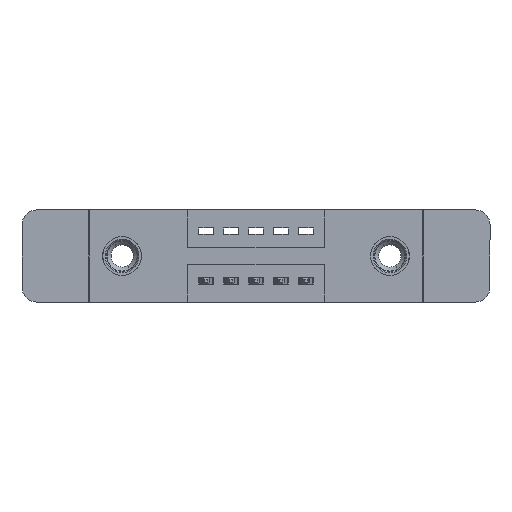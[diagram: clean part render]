
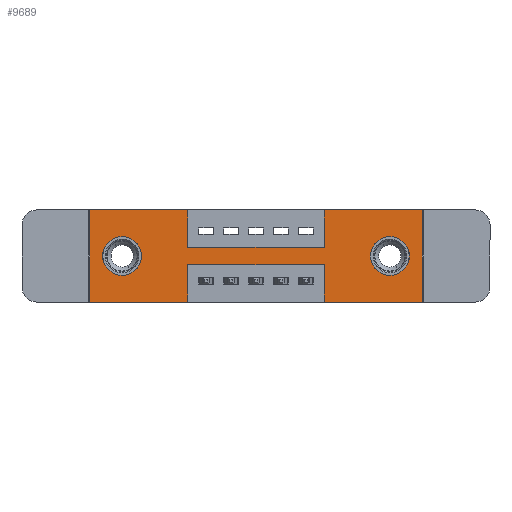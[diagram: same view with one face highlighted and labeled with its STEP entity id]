
A CAD part, front view. The second image highlights one B-rep face of the part: STEP entity #9689.
In plain terms, the highlighted planar face has unit normal (0, -1, 0).
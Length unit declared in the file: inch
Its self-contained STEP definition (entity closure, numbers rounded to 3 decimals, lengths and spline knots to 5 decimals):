
#65 = ORIENTED_EDGE ( 'NONE', *, *, #8855, .F. ) ;
#238 = CARTESIAN_POINT ( 'NONE',  ( 0.3925, 0., -0.15 ) ) ;
#316 = EDGE_CURVE ( 'NONE', #12437, #9325, #3677, .T. ) ;
#398 = CARTESIAN_POINT ( 'NONE',  ( 0.13, 0., -0.107 ) ) ;
#513 = ORIENTED_EDGE ( 'NONE', *, *, #13121, .F. ) ;
#515 = DIRECTION ( 'NONE',  ( 0., -1., 0. ) ) ;
#548 = AXIS2_PLACEMENT_3D ( 'NONE', #12380, #5952, #3836 ) ;
#571 = DIRECTION ( 'NONE',  ( 0., 0., -1. ) ) ;
#589 = CARTESIAN_POINT ( 'NONE',  ( 0., 0., -0.37 ) ) ;
#710 = VERTEX_POINT ( 'NONE', #9934 ) ;
#1002 = FACE_BOUND ( 'NONE', #13647, .T. ) ;
#1072 = VECTOR ( 'NONE', #3995, 39.37008 ) ;
#1135 = EDGE_CURVE ( 'NONE', #1375, #8630, #1816, .T. ) ;
#1375 = VERTEX_POINT ( 'NONE', #13892 ) ;
#1467 = CARTESIAN_POINT ( 'NONE',  ( 0., 0., 0. ) ) ;
#1702 = VERTEX_POINT ( 'NONE', #7145 ) ;
#1800 = CARTESIAN_POINT ( 'NONE',  ( 0., 0., -0.37 ) ) ;
#1816 = LINE ( 'NONE', #9152, #13083 ) ;
#1893 = CIRCLE ( 'NONE', #8534, 0.078 ) ;
#1899 = ORIENTED_EDGE ( 'NONE', *, *, #11169, .F. ) ;
#1965 = CARTESIAN_POINT ( 'NONE',  ( 0., 0., 0. ) ) ;
#1981 = CARTESIAN_POINT ( 'NONE',  ( 0.3925, 0., -0.37 ) ) ;
#2000 = CARTESIAN_POINT ( 'NONE',  ( 0.3925, 0., 0. ) ) ;
#2028 = ORIENTED_EDGE ( 'NONE', *, *, #316, .T. ) ;
#2043 = ORIENTED_EDGE ( 'NONE', *, *, #1135, .F. ) ;
#2092 = DIRECTION ( 'NONE',  ( 0., 0., -1. ) ) ;
#2189 = VERTEX_POINT ( 'NONE', #7234 ) ;
#2314 = CARTESIAN_POINT ( 'NONE',  ( 0., 0., 0. ) ) ;
#2426 = VECTOR ( 'NONE', #8026, 39.37008 ) ;
#2436 = EDGE_CURVE ( 'NONE', #1702, #11896, #8684, .T. ) ;
#2542 = EDGE_CURVE ( 'NONE', #710, #1375, #6013, .T. ) ;
#2558 = CIRCLE ( 'NONE', #548, 0.078 ) ;
#2663 = PLANE ( 'NONE',  #7568 ) ;
#2978 = VERTEX_POINT ( 'NONE', #398 ) ;
#3062 = ORIENTED_EDGE ( 'NONE', *, *, #13079, .F. ) ;
#3138 = DIRECTION ( 'NONE',  ( 0., 0., -1. ) ) ;
#3182 = VERTEX_POINT ( 'NONE', #5188 ) ;
#3246 = VECTOR ( 'NONE', #9193, 39.37008 ) ;
#3677 = CIRCLE ( 'NONE', #13862, 0.078 ) ;
#3764 = CARTESIAN_POINT ( 'NONE',  ( 0., 0., -0.37 ) ) ;
#3794 = CARTESIAN_POINT ( 'NONE',  ( 0.9425, 0., 0. ) ) ;
#3815 = CARTESIAN_POINT ( 'NONE',  ( 1.205, 0., -0.185 ) ) ;
#3836 = DIRECTION ( 'NONE',  ( 0., 0., 1. ) ) ;
#3938 = CIRCLE ( 'NONE', #5187, 0.078 ) ;
#3967 = CARTESIAN_POINT ( 'NONE',  ( 0.3925, 0., -0.22 ) ) ;
#3990 = LINE ( 'NONE', #2314, #9192 ) ;
#3995 = DIRECTION ( 'NONE',  ( -1., 0., 0. ) ) ;
#3996 = VERTEX_POINT ( 'NONE', #12141 ) ;
#4077 = EDGE_CURVE ( 'NONE', #13248, #2978, #2558, .T. ) ;
#4109 = VECTOR ( 'NONE', #4788, 39.37008 ) ;
#4272 = EDGE_CURVE ( 'NONE', #2978, #13248, #1893, .T. ) ;
#4352 = EDGE_CURVE ( 'NONE', #9325, #12437, #3938, .T. ) ;
#4690 = VECTOR ( 'NONE', #12716, 39.37008 ) ;
#4745 = CARTESIAN_POINT ( 'NONE',  ( 0.13, 0., -0.185 ) ) ;
#4788 = DIRECTION ( 'NONE',  ( 0., 0., 1. ) ) ;
#4891 = DIRECTION ( 'NONE',  ( 0., 1., 0. ) ) ;
#4926 = CARTESIAN_POINT ( 'NONE',  ( 1.205, 0., -0.185 ) ) ;
#4978 = VECTOR ( 'NONE', #9907, 39.37008 ) ;
#5187 = AXIS2_PLACEMENT_3D ( 'NONE', #3815, #4891, #571 ) ;
#5188 = CARTESIAN_POINT ( 'NONE',  ( 0.3925, 0., -0.15 ) ) ;
#5259 = EDGE_CURVE ( 'NONE', #6263, #3996, #8949, .T. ) ;
#5319 = CARTESIAN_POINT ( 'NONE',  ( 0.9425, 0., -0.22 ) ) ;
#5565 = ORIENTED_EDGE ( 'NONE', *, *, #10179, .F. ) ;
#5586 = FACE_BOUND ( 'NONE', #8133, .T. ) ;
#5814 = CARTESIAN_POINT ( 'NONE',  ( 1.205, 0., -0.263 ) ) ;
#5893 = ORIENTED_EDGE ( 'NONE', *, *, #8638, .F. ) ;
#5895 = DIRECTION ( 'NONE',  ( 0., 0., 1. ) ) ;
#5952 = DIRECTION ( 'NONE',  ( 0., 1., 0. ) ) ;
#6013 = LINE ( 'NONE', #1800, #1072 ) ;
#6119 = LINE ( 'NONE', #10187, #3246 ) ;
#6263 = VERTEX_POINT ( 'NONE', #3967 ) ;
#6679 = CARTESIAN_POINT ( 'NONE',  ( 0., 0., -0.37 ) ) ;
#6741 = VECTOR ( 'NONE', #9300, 39.37008 ) ;
#6863 = DIRECTION ( 'NONE',  ( 0., 1., 0. ) ) ;
#6876 = DIRECTION ( 'NONE',  ( -1., 0., 0. ) ) ;
#6900 = DIRECTION ( 'NONE',  ( 0., 0., 1. ) ) ;
#6904 = DIRECTION ( 'NONE',  ( 1., 0., 0. ) ) ;
#7086 = DIRECTION ( 'NONE',  ( 0., 1., 0. ) ) ;
#7113 = LINE ( 'NONE', #1467, #4109 ) ;
#7145 = CARTESIAN_POINT ( 'NONE',  ( 0.9425, 0., -0.15 ) ) ;
#7234 = CARTESIAN_POINT ( 'NONE',  ( 0.3925, 0., 0. ) ) ;
#7275 = LINE ( 'NONE', #589, #8781 ) ;
#7568 = AXIS2_PLACEMENT_3D ( 'NONE', #3764, #515, #13416 ) ;
#7748 = LINE ( 'NONE', #238, #6741 ) ;
#7854 = VERTEX_POINT ( 'NONE', #1965 ) ;
#8026 = DIRECTION ( 'NONE',  ( 0., 0., 1. ) ) ;
#8059 = EDGE_CURVE ( 'NONE', #11896, #13049, #6119, .T. ) ;
#8133 = EDGE_LOOP ( 'NONE', ( #2028, #12892 ) ) ;
#8154 = VECTOR ( 'NONE', #2092, 39.37008 ) ;
#8534 = AXIS2_PLACEMENT_3D ( 'NONE', #4745, #6863, #5895 ) ;
#8630 = VERTEX_POINT ( 'NONE', #5319 ) ;
#8638 = EDGE_CURVE ( 'NONE', #2189, #3182, #8640, .T. ) ;
#8640 = LINE ( 'NONE', #2000, #8154 ) ;
#8684 = LINE ( 'NONE', #9249, #2426 ) ;
#8781 = VECTOR ( 'NONE', #6876, 39.37008 ) ;
#8855 = EDGE_CURVE ( 'NONE', #10774, #7854, #7113, .T. ) ;
#8949 = LINE ( 'NONE', #1981, #10474 ) ;
#8993 = ORIENTED_EDGE ( 'NONE', *, *, #5259, .F. ) ;
#9152 = CARTESIAN_POINT ( 'NONE',  ( 0.9425, 0., -0.37 ) ) ;
#9192 = VECTOR ( 'NONE', #6904, 39.37008 ) ;
#9193 = DIRECTION ( 'NONE',  ( 1., 0., 0. ) ) ;
#9249 = CARTESIAN_POINT ( 'NONE',  ( 0.9425, 0., 0. ) ) ;
#9281 = EDGE_CURVE ( 'NONE', #3996, #10774, #7275, .T. ) ;
#9300 = DIRECTION ( 'NONE',  ( 1., 0., 0. ) ) ;
#9325 = VERTEX_POINT ( 'NONE', #5814 ) ;
#9689 = ADVANCED_FACE ( 'NONE', ( #5586, #1002, #10470 ), #2663, .T. ) ;
#9907 = DIRECTION ( 'NONE',  ( -1., 0., 0. ) ) ;
#9934 = CARTESIAN_POINT ( 'NONE',  ( 1.335, 0., -0.37 ) ) ;
#10179 = EDGE_CURVE ( 'NONE', #3182, #1702, #7748, .T. ) ;
#10187 = CARTESIAN_POINT ( 'NONE',  ( 0., 0., 0. ) ) ;
#10272 = ORIENTED_EDGE ( 'NONE', *, *, #8059, .F. ) ;
#10434 = CARTESIAN_POINT ( 'NONE',  ( 1.335, 0., 0. ) ) ;
#10470 = FACE_OUTER_BOUND ( 'NONE', #13195, .T. ) ;
#10474 = VECTOR ( 'NONE', #3138, 39.37008 ) ;
#10565 = ORIENTED_EDGE ( 'NONE', *, *, #4077, .T. ) ;
#10641 = ORIENTED_EDGE ( 'NONE', *, *, #4272, .T. ) ;
#10774 = VERTEX_POINT ( 'NONE', #6679 ) ;
#10840 = CARTESIAN_POINT ( 'NONE',  ( 0.3925, 0., -0.22 ) ) ;
#11169 = EDGE_CURVE ( 'NONE', #13049, #710, #13924, .T. ) ;
#11468 = ORIENTED_EDGE ( 'NONE', *, *, #2542, .F. ) ;
#11896 = VERTEX_POINT ( 'NONE', #3794 ) ;
#12046 = LINE ( 'NONE', #10840, #4978 ) ;
#12074 = CARTESIAN_POINT ( 'NONE',  ( 1.335, 0., 0. ) ) ;
#12141 = CARTESIAN_POINT ( 'NONE',  ( 0.3925, 0., -0.37 ) ) ;
#12353 = CARTESIAN_POINT ( 'NONE',  ( 0.13, 0., -0.263 ) ) ;
#12356 = DIRECTION ( 'NONE',  ( 0., 0., -1. ) ) ;
#12380 = CARTESIAN_POINT ( 'NONE',  ( 0.13, 0., -0.185 ) ) ;
#12437 = VERTEX_POINT ( 'NONE', #12441 ) ;
#12441 = CARTESIAN_POINT ( 'NONE',  ( 1.205, 0., -0.107 ) ) ;
#12716 = DIRECTION ( 'NONE',  ( 0., 0., -1. ) ) ;
#12735 = ORIENTED_EDGE ( 'NONE', *, *, #2436, .F. ) ;
#12892 = ORIENTED_EDGE ( 'NONE', *, *, #4352, .T. ) ;
#13049 = VERTEX_POINT ( 'NONE', #12074 ) ;
#13079 = EDGE_CURVE ( 'NONE', #8630, #6263, #12046, .T. ) ;
#13083 = VECTOR ( 'NONE', #6900, 39.37008 ) ;
#13121 = EDGE_CURVE ( 'NONE', #7854, #2189, #3990, .T. ) ;
#13195 = EDGE_LOOP ( 'NONE', ( #8993, #3062, #2043, #11468, #1899, #10272, #12735, #5565, #5893, #513, #65, #13818 ) ) ;
#13248 = VERTEX_POINT ( 'NONE', #12353 ) ;
#13416 = DIRECTION ( 'NONE',  ( 0., 0., -1. ) ) ;
#13647 = EDGE_LOOP ( 'NONE', ( #10641, #10565 ) ) ;
#13818 = ORIENTED_EDGE ( 'NONE', *, *, #9281, .F. ) ;
#13862 = AXIS2_PLACEMENT_3D ( 'NONE', #4926, #7086, #12356 ) ;
#13892 = CARTESIAN_POINT ( 'NONE',  ( 0.9425, 0., -0.37 ) ) ;
#13924 = LINE ( 'NONE', #10434, #4690 ) ;
